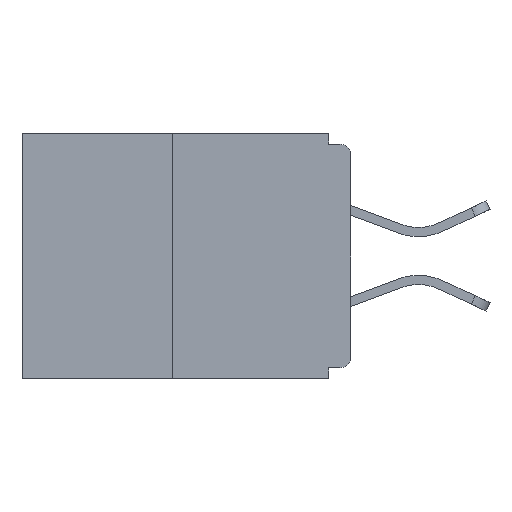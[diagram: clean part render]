
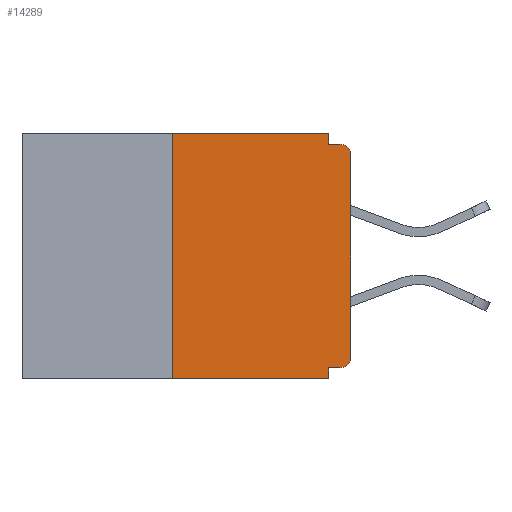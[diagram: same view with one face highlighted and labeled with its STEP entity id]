
A CAD part, left-side view. The second image highlights one B-rep face of the part: STEP entity #14289.
In plain terms, the highlighted planar face has unit normal (-1, 0, 0).
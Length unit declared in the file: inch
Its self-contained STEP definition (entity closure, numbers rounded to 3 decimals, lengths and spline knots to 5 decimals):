
#7 = VECTOR ( 'NONE', #3763, 39.37008 ) ;
#131 = LINE ( 'NONE', #7203, #7 ) ;
#490 = VERTEX_POINT ( 'NONE', #5671 ) ;
#543 = EDGE_CURVE ( 'NONE', #17064, #15796, #20789, .T. ) ;
#739 = DIRECTION ( 'NONE',  ( 0., 0., -1. ) ) ;
#751 = ORIENTED_EDGE ( 'NONE', *, *, #17591, .F. ) ;
#1351 = VERTEX_POINT ( 'NONE', #4116 ) ;
#1402 = AXIS2_PLACEMENT_3D ( 'NONE', #2605, #20348, #739 ) ;
#1516 = ORIENTED_EDGE ( 'NONE', *, *, #543, .F. ) ;
#1750 = DIRECTION ( 'NONE',  ( 0., 0., 1. ) ) ;
#1811 = DIRECTION ( 'NONE',  ( -1., 0., 0. ) ) ;
#1912 = VECTOR ( 'NONE', #7716, 39.37008 ) ;
#2605 = CARTESIAN_POINT ( 'NONE',  ( 0., 0.015, -0.313 ) ) ;
#2791 = VERTEX_POINT ( 'NONE', #9374 ) ;
#2935 = DIRECTION ( 'NONE',  ( 0., -1., 0. ) ) ;
#3065 = LINE ( 'NONE', #3171, #10346 ) ;
#3171 = CARTESIAN_POINT ( 'NONE',  ( 0., 0.031, 0. ) ) ;
#3236 = ORIENTED_EDGE ( 'NONE', *, *, #21701, .T. ) ;
#3303 = FACE_OUTER_BOUND ( 'NONE', #12122, .T. ) ;
#3426 = PLANE ( 'NONE',  #8457 ) ;
#3763 = DIRECTION ( 'NONE',  ( 0., 1., 0. ) ) ;
#3862 = LINE ( 'NONE', #21716, #5447 ) ;
#4116 = CARTESIAN_POINT ( 'NONE',  ( 0., 0.031, -0.343 ) ) ;
#4404 = LINE ( 'NONE', #11502, #21224 ) ;
#5447 = VECTOR ( 'NONE', #8881, 39.37008 ) ;
#5671 = CARTESIAN_POINT ( 'NONE',  ( 0., 0.031, -0.328 ) ) ;
#6023 = LINE ( 'NONE', #11782, #15843 ) ;
#6681 = CARTESIAN_POINT ( 'NONE',  ( 0., 0.015, -0.328 ) ) ;
#6935 = CIRCLE ( 'NONE', #1402, 0.015 ) ;
#7170 = LINE ( 'NONE', #21257, #10780 ) ;
#7203 = CARTESIAN_POINT ( 'NONE',  ( 0., 0., -0.328 ) ) ;
#7207 = EDGE_CURVE ( 'NONE', #14660, #17064, #3065, .T. ) ;
#7716 = DIRECTION ( 'NONE',  ( 0., -1., 0. ) ) ;
#7962 = EDGE_CURVE ( 'NONE', #490, #1351, #4404, .T. ) ;
#8017 = LINE ( 'NONE', #15520, #23066 ) ;
#8457 = AXIS2_PLACEMENT_3D ( 'NONE', #17578, #12164, #15549 ) ;
#8568 = CARTESIAN_POINT ( 'NONE',  ( 0., 0.015, -0.03 ) ) ;
#8881 = DIRECTION ( 'NONE',  ( 0., -1., 0. ) ) ;
#8989 = CARTESIAN_POINT ( 'NONE',  ( 0., 0.015, -0.015 ) ) ;
#9056 = CARTESIAN_POINT ( 'NONE',  ( 0., 0.25, 0. ) ) ;
#9374 = CARTESIAN_POINT ( 'NONE',  ( 0., 0.25, -0.343 ) ) ;
#9503 = VERTEX_POINT ( 'NONE', #6681 ) ;
#9790 = DIRECTION ( 'NONE',  ( 0., 0., 1. ) ) ;
#10151 = CARTESIAN_POINT ( 'NONE',  ( 0., 0., -0.313 ) ) ;
#10270 = DIRECTION ( 'NONE',  ( 0., 0., -1. ) ) ;
#10346 = VECTOR ( 'NONE', #10270, 39.37008 ) ;
#10480 = ORIENTED_EDGE ( 'NONE', *, *, #14207, .T. ) ;
#10780 = VECTOR ( 'NONE', #1750, 39.37008 ) ;
#11442 = ORIENTED_EDGE ( 'NONE', *, *, #17141, .F. ) ;
#11502 = CARTESIAN_POINT ( 'NONE',  ( 0., 0.031, -0.343 ) ) ;
#11688 = ORIENTED_EDGE ( 'NONE', *, *, #14453, .T. ) ;
#11782 = CARTESIAN_POINT ( 'NONE',  ( 0., 0., 0. ) ) ;
#11850 = EDGE_CURVE ( 'NONE', #22598, #19192, #6023, .T. ) ;
#11873 = CARTESIAN_POINT ( 'NONE',  ( 0., 0.031, 0. ) ) ;
#12122 = EDGE_LOOP ( 'NONE', ( #751, #11442, #11688, #22060, #15630, #10480, #20208, #3236, #1516, #12277 ) ) ;
#12164 = DIRECTION ( 'NONE',  ( 1., 0., 0. ) ) ;
#12277 = ORIENTED_EDGE ( 'NONE', *, *, #7207, .F. ) ;
#13075 = VERTEX_POINT ( 'NONE', #9056 ) ;
#13534 = AXIS2_PLACEMENT_3D ( 'NONE', #8568, #1811, #19216 ) ;
#14207 = EDGE_CURVE ( 'NONE', #9503, #22598, #6935, .T. ) ;
#14289 = ADVANCED_FACE ( 'NONE', ( #3303 ), #3426, .F. ) ;
#14453 = EDGE_CURVE ( 'NONE', #2791, #1351, #3862, .T. ) ;
#14660 = VERTEX_POINT ( 'NONE', #11873 ) ;
#15396 = CIRCLE ( 'NONE', #13534, 0.015 ) ;
#15520 = CARTESIAN_POINT ( 'NONE',  ( 0., 0.46, 0. ) ) ;
#15549 = DIRECTION ( 'NONE',  ( 0., 0., -1. ) ) ;
#15630 = ORIENTED_EDGE ( 'NONE', *, *, #17098, .F. ) ;
#15796 = VERTEX_POINT ( 'NONE', #8989 ) ;
#15843 = VECTOR ( 'NONE', #9790, 39.37008 ) ;
#16639 = CARTESIAN_POINT ( 'NONE',  ( 0., 0., -0.015 ) ) ;
#16755 = CARTESIAN_POINT ( 'NONE',  ( 0., 0., -0.03 ) ) ;
#17064 = VERTEX_POINT ( 'NONE', #21721 ) ;
#17098 = EDGE_CURVE ( 'NONE', #9503, #490, #131, .T. ) ;
#17141 = EDGE_CURVE ( 'NONE', #2791, #13075, #7170, .T. ) ;
#17578 = CARTESIAN_POINT ( 'NONE',  ( 0., 0.46, 0. ) ) ;
#17591 = EDGE_CURVE ( 'NONE', #13075, #14660, #8017, .T. ) ;
#18657 = DIRECTION ( 'NONE',  ( 0., 0., -1. ) ) ;
#19192 = VERTEX_POINT ( 'NONE', #16755 ) ;
#19216 = DIRECTION ( 'NONE',  ( 0., 0., -1. ) ) ;
#20208 = ORIENTED_EDGE ( 'NONE', *, *, #11850, .T. ) ;
#20348 = DIRECTION ( 'NONE',  ( -1., 0., 0. ) ) ;
#20789 = LINE ( 'NONE', #16639, #1912 ) ;
#21224 = VECTOR ( 'NONE', #18657, 39.37008 ) ;
#21257 = CARTESIAN_POINT ( 'NONE',  ( 0., 0.25, 0. ) ) ;
#21701 = EDGE_CURVE ( 'NONE', #19192, #15796, #15396, .T. ) ;
#21716 = CARTESIAN_POINT ( 'NONE',  ( 0., 0.46, -0.343 ) ) ;
#21721 = CARTESIAN_POINT ( 'NONE',  ( 0., 0.031, -0.015 ) ) ;
#22060 = ORIENTED_EDGE ( 'NONE', *, *, #7962, .F. ) ;
#22598 = VERTEX_POINT ( 'NONE', #10151 ) ;
#23066 = VECTOR ( 'NONE', #2935, 39.37008 ) ;
